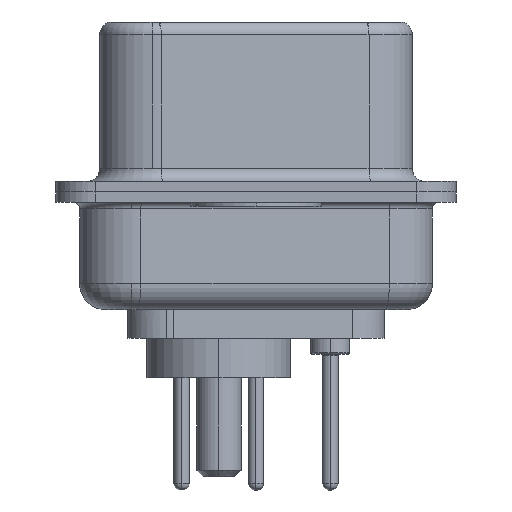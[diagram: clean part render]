
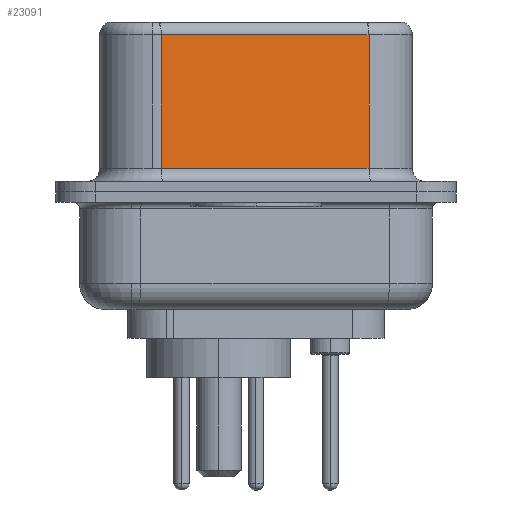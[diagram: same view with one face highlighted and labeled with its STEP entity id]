
A CAD part, left-side view. The second image highlights one B-rep face of the part: STEP entity #23091.
In plain terms, the highlighted planar face has unit normal (-0.985, -0.174, 0).
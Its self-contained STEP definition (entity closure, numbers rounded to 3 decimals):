
#344 = LINE ( 'NONE', #4536, #14689 ) ;
#757 = ORIENTED_EDGE ( 'NONE', *, *, #6520, .T. ) ;
#1418 = DIRECTION ( 'NONE',  ( -0.174, 0.985, 0. ) ) ;
#1708 = DIRECTION ( 'NONE',  ( 0., 0., -1. ) ) ;
#2877 = ORIENTED_EDGE ( 'NONE', *, *, #7976, .F. ) ;
#3102 = FACE_OUTER_BOUND ( 'NONE', #17983, .T. ) ;
#3907 = VERTEX_POINT ( 'NONE', #16442 ) ;
#4536 = CARTESIAN_POINT ( 'NONE',  ( 5.132, -4.322, 0.9 ) ) ;
#5476 = CARTESIAN_POINT ( 'NONE',  ( 5.132, -4.322, 6.52 ) ) ;
#6520 = EDGE_CURVE ( 'NONE', #3907, #22514, #8167, .T. ) ;
#6789 = ORIENTED_EDGE ( 'NONE', *, *, #9561, .T. ) ;
#6989 = VERTEX_POINT ( 'NONE', #24032 ) ;
#7976 = EDGE_CURVE ( 'NONE', #15155, #6989, #18986, .T. ) ;
#8167 = LINE ( 'NONE', #19777, #12551 ) ;
#9184 = DIRECTION ( 'NONE',  ( -0.174, 0.985, 0. ) ) ;
#9561 = EDGE_CURVE ( 'NONE', #22514, #6989, #344, .T. ) ;
#10600 = CARTESIAN_POINT ( 'NONE',  ( 5.132, -4.322, 6.02 ) ) ;
#12551 = VECTOR ( 'NONE', #19450, 1000. ) ;
#12565 = PLANE ( 'NONE',  #23853 ) ;
#12644 = DIRECTION ( 'NONE',  ( 0.985, 0.174, 0. ) ) ;
#14526 = CARTESIAN_POINT ( 'NONE',  ( 3.73, 3.628, 0.9 ) ) ;
#14689 = VECTOR ( 'NONE', #21424, 1000. ) ;
#15155 = VERTEX_POINT ( 'NONE', #10600 ) ;
#16442 = CARTESIAN_POINT ( 'NONE',  ( 3.73, 3.628, 6.02 ) ) ;
#16645 = ORIENTED_EDGE ( 'NONE', *, *, #23789, .T. ) ;
#17983 = EDGE_LOOP ( 'NONE', ( #2877, #16645, #757, #6789 ) ) ;
#18986 = LINE ( 'NONE', #5476, #23509 ) ;
#19450 = DIRECTION ( 'NONE',  ( 0., 0., -1. ) ) ;
#19522 = VECTOR ( 'NONE', #9184, 1000. ) ;
#19777 = CARTESIAN_POINT ( 'NONE',  ( 3.73, 3.628, 6.52 ) ) ;
#20124 = LINE ( 'NONE', #24359, #19522 ) ;
#20145 = CARTESIAN_POINT ( 'NONE',  ( 5.132, -4.322, 6.52 ) ) ;
#21424 = DIRECTION ( 'NONE',  ( 0.174, -0.985, 0. ) ) ;
#22514 = VERTEX_POINT ( 'NONE', #14526 ) ;
#23091 = ADVANCED_FACE ( 'NONE', ( #3102 ), #12565, .F. ) ;
#23509 = VECTOR ( 'NONE', #1708, 1000. ) ;
#23789 = EDGE_CURVE ( 'NONE', #15155, #3907, #20124, .T. ) ;
#23853 = AXIS2_PLACEMENT_3D ( 'NONE', #20145, #12644, #1418 ) ;
#24032 = CARTESIAN_POINT ( 'NONE',  ( 5.132, -4.322, 0.9 ) ) ;
#24359 = CARTESIAN_POINT ( 'NONE',  ( 5.132, -4.322, 6.02 ) ) ;
